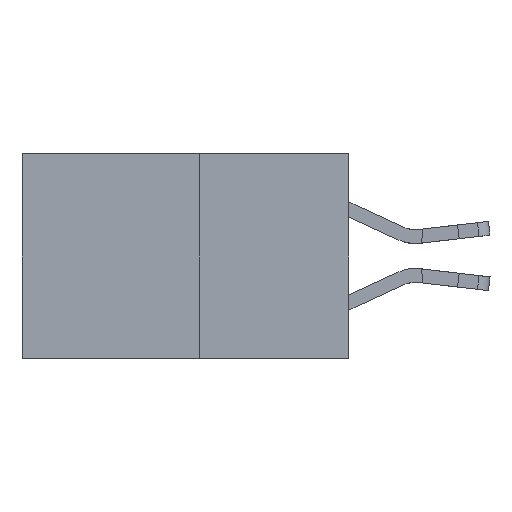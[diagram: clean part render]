
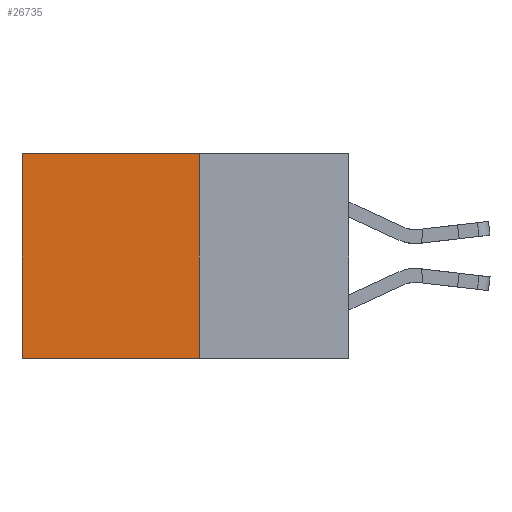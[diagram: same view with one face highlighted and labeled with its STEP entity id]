
A CAD part, left-side view. The second image highlights one B-rep face of the part: STEP entity #26735.
In plain terms, the highlighted planar face has unit normal (-1, 0, 0).
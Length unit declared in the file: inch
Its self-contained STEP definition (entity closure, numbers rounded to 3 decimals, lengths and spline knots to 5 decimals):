
#472 = DIRECTION ( 'NONE',  ( 0., 1., 0. ) ) ;
#579 = ORIENTED_EDGE ( 'NONE', *, *, #1147, .F. ) ;
#611 = VERTEX_POINT ( 'NONE', #4924 ) ;
#1147 = EDGE_CURVE ( 'NONE', #611, #3864, #13126, .T. ) ;
#2269 = PLANE ( 'NONE',  #18740 ) ;
#3440 = LINE ( 'NONE', #14740, #16676 ) ;
#3864 = VERTEX_POINT ( 'NONE', #6069 ) ;
#4509 = DIRECTION ( 'NONE',  ( 0., 1., 0. ) ) ;
#4924 = CARTESIAN_POINT ( 'NONE',  ( 0.277, 0.27, 0. ) ) ;
#6069 = CARTESIAN_POINT ( 'NONE',  ( 0.277, 0.27, -0.37 ) ) ;
#7180 = DIRECTION ( 'NONE',  ( 1., 0., 0. ) ) ;
#7496 = VERTEX_POINT ( 'NONE', #27561 ) ;
#12190 = DIRECTION ( 'NONE',  ( 0., 0., -1. ) ) ;
#12533 = FACE_OUTER_BOUND ( 'NONE', #17581, .T. ) ;
#13126 = LINE ( 'NONE', #24889, #18549 ) ;
#13733 = LINE ( 'NONE', #13868, #18419 ) ;
#13868 = CARTESIAN_POINT ( 'NONE',  ( 0.277, 0.27, -0.37 ) ) ;
#14480 = EDGE_CURVE ( 'NONE', #611, #22715, #3440, .T. ) ;
#14740 = CARTESIAN_POINT ( 'NONE',  ( 0.277, 0.27, 0. ) ) ;
#15493 = EDGE_CURVE ( 'NONE', #3864, #7496, #13733, .T. ) ;
#16676 = VECTOR ( 'NONE', #472, 39.37008 ) ;
#16752 = CARTESIAN_POINT ( 'NONE',  ( 0.277, 0.59, -0.37 ) ) ;
#17404 = VECTOR ( 'NONE', #12190, 39.37008 ) ;
#17581 = EDGE_LOOP ( 'NONE', ( #28790, #25584, #579, #20152 ) ) ;
#18419 = VECTOR ( 'NONE', #4509, 39.37008 ) ;
#18549 = VECTOR ( 'NONE', #21420, 39.37008 ) ;
#18740 = AXIS2_PLACEMENT_3D ( 'NONE', #21121, #7180, #23490 ) ;
#20152 = ORIENTED_EDGE ( 'NONE', *, *, #14480, .T. ) ;
#21121 = CARTESIAN_POINT ( 'NONE',  ( 0.277, 0.27, -0.37 ) ) ;
#21420 = DIRECTION ( 'NONE',  ( 0., 0., -1. ) ) ;
#22715 = VERTEX_POINT ( 'NONE', #29736 ) ;
#23490 = DIRECTION ( 'NONE',  ( 0., 0., -1. ) ) ;
#23650 = LINE ( 'NONE', #16752, #17404 ) ;
#24237 = EDGE_CURVE ( 'NONE', #22715, #7496, #23650, .T. ) ;
#24889 = CARTESIAN_POINT ( 'NONE',  ( 0.277, 0.27, -0.37 ) ) ;
#25584 = ORIENTED_EDGE ( 'NONE', *, *, #15493, .F. ) ;
#26735 = ADVANCED_FACE ( 'NONE', ( #12533 ), #2269, .F. ) ;
#27561 = CARTESIAN_POINT ( 'NONE',  ( 0.277, 0.59, -0.37 ) ) ;
#28790 = ORIENTED_EDGE ( 'NONE', *, *, #24237, .T. ) ;
#29736 = CARTESIAN_POINT ( 'NONE',  ( 0.277, 0.59, 0. ) ) ;
